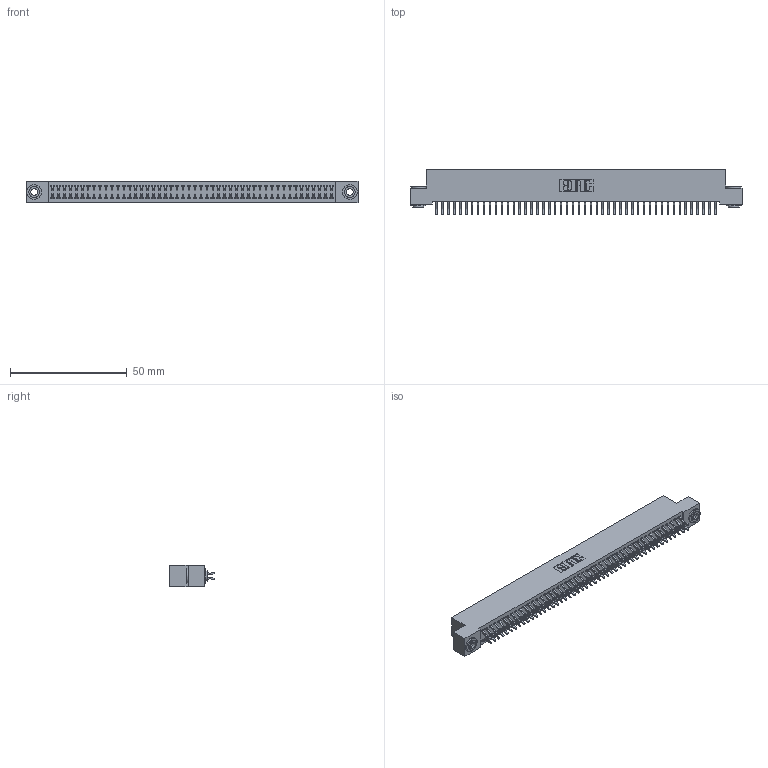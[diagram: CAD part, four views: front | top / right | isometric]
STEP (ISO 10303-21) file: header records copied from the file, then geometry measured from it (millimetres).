
FILE_DESCRIPTION (( 'STEP AP203' ), '1' );
FILE_NAME ('392-096-556-203.STEP', '2018-08-18T10:12:54', ( '' ), ( '' ), 'SwSTEP 2.0', 'SolidWorks 2016', '' );
FILE_SCHEMA (( 'CONFIG_CONTROL_DESIGN' ));
Length unit declared in the file: inch
Products named in the file (4): 342 Part_.156 TH; 345-292-001_556 Tail; 342-250-002_345-250-002-102; 392-096-556-203
Assembly tree (99 placements, depth 2):
  392-096-556-203
    342 Part_.156 TH
    345-292-001_556 Tail  x96
    342-250-002_345-250-002-102  x2
Bounding box: 142.24 x 19.58 x 9.4 mm (x, y, z)
Volume: 12829 mm3; surface area: 21151.2 mm2
Topology: 99 solids, 99 shells, 5716 faces, 16983 edges, 11190 vertices
Faces by surface type: plane 3916, cylinder 1792, cone 8
Entity records: 30842 total; most frequent: CARTESIAN_POINT 5093, ORIENTED_EDGE 5010, DIRECTION 4363, EDGE_CURVE 2505, VECTOR 2345, LINE 2345, VERTEX_POINT 1666, AXIS2_PLACEMENT_3D 1009
